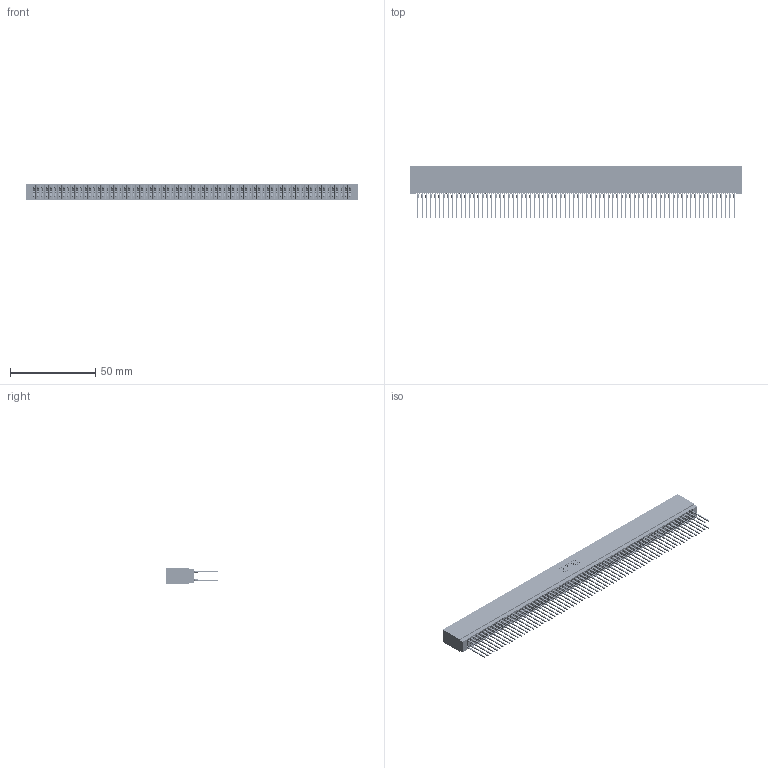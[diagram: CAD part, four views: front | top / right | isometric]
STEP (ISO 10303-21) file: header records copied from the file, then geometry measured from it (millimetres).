
FILE_DESCRIPTION (( 'STEP AP203' ), '1' );
FILE_NAME ('745-148-540-201.STEP', '2020-09-15T13:30:16', ( '' ), ( '' ), 'SwSTEP 2.0', 'SolidWorks 2020', '' );
FILE_SCHEMA (( 'CONFIG_CONTROL_DESIGN' ));
Products named in the file (3): 745-292-001_540; 745-148-540-201; 745 Part_Insulator Option - 01
Assembly tree (149 placements, depth 2):
  745-148-540-201
    745 Part_Insulator Option - 01
    745-292-001_540  x148
Bounding box: 194.56 x 30.62 x 8.89 mm (x, y, z)
Volume: 17766.1 mm3; surface area: 38566.2 mm2
Topology: 149 solids, 149 shells, 13341 faces, 35852 edges, 22520 vertices
Faces by surface type: plane 6863, bspline 2960, cylinder 2630, torus 888
Entity records: 120218 total; most frequent: CARTESIAN_POINT 21343, ORIENTED_EDGE 20842, DIRECTION 18179, EDGE_CURVE 10421, VECTOR 9795, LINE 9795, VERTEX_POINT 6644, AXIS2_PLACEMENT_3D 4192
